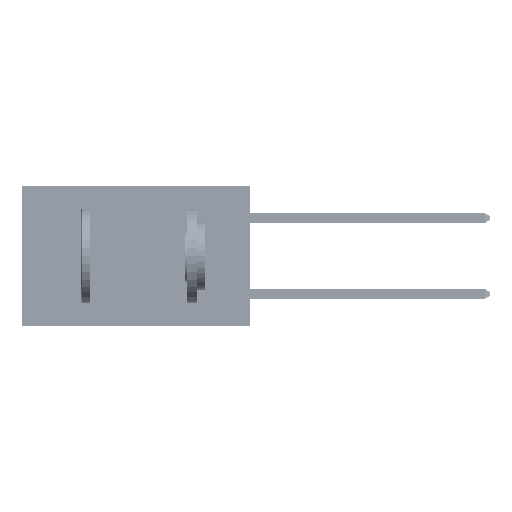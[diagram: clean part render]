
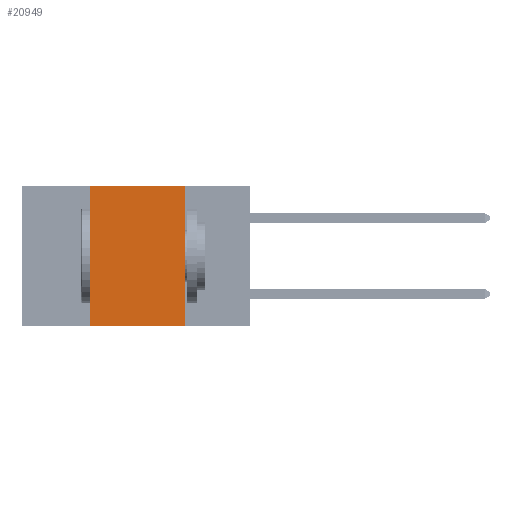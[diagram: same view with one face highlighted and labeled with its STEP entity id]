
A CAD part, left-side view. The second image highlights one B-rep face of the part: STEP entity #20949.
In plain terms, the highlighted planar face has unit normal (-1, 0, 0).
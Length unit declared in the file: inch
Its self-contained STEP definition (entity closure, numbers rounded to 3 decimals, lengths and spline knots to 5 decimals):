
#704 = VECTOR ( 'NONE', #45560, 39.37008 ) ;
#7364 = CARTESIAN_POINT ( 'NONE',  ( 0., 0.6, 0. ) ) ;
#10146 = CARTESIAN_POINT ( 'NONE',  ( 0., 0.17, 0. ) ) ;
#11163 = VERTEX_POINT ( 'NONE', #21826 ) ;
#11632 = AXIS2_PLACEMENT_3D ( 'NONE', #7364, #15367, #20673 ) ;
#12358 = LINE ( 'NONE', #42086, #704 ) ;
#12411 = EDGE_CURVE ( 'NONE', #17411, #30723, #38642, .T. ) ;
#13023 = DIRECTION ( 'NONE',  ( 0., -1., 0. ) ) ;
#13771 = EDGE_LOOP ( 'NONE', ( #38287, #25829, #31517, #31889 ) ) ;
#14412 = LINE ( 'NONE', #19038, #44380 ) ;
#15367 = DIRECTION ( 'NONE',  ( 1., 0., 0. ) ) ;
#16229 = EDGE_CURVE ( 'NONE', #17411, #11163, #12358, .T. ) ;
#16359 = VERTEX_POINT ( 'NONE', #49490 ) ;
#17411 = VERTEX_POINT ( 'NONE', #23085 ) ;
#19038 = CARTESIAN_POINT ( 'NONE',  ( 0., 0.6, 0. ) ) ;
#20673 = DIRECTION ( 'NONE',  ( 0., 0., -1. ) ) ;
#20723 = CARTESIAN_POINT ( 'NONE',  ( 0., 0.6, -0.37 ) ) ;
#20949 = ADVANCED_FACE ( 'NONE', ( #33537 ), #26985, .F. ) ;
#21826 = CARTESIAN_POINT ( 'NONE',  ( 0., 0.42, 0. ) ) ;
#23085 = CARTESIAN_POINT ( 'NONE',  ( 0., 0.42, -0.37 ) ) ;
#25829 = ORIENTED_EDGE ( 'NONE', *, *, #42701, .F. ) ;
#26985 = PLANE ( 'NONE',  #11632 ) ;
#27587 = LINE ( 'NONE', #10146, #44094 ) ;
#30723 = VERTEX_POINT ( 'NONE', #49356 ) ;
#31517 = ORIENTED_EDGE ( 'NONE', *, *, #16229, .F. ) ;
#31889 = ORIENTED_EDGE ( 'NONE', *, *, #12411, .T. ) ;
#33537 = FACE_OUTER_BOUND ( 'NONE', #13771, .T. ) ;
#38287 = ORIENTED_EDGE ( 'NONE', *, *, #45279, .F. ) ;
#38642 = LINE ( 'NONE', #20723, #46609 ) ;
#42086 = CARTESIAN_POINT ( 'NONE',  ( 0., 0.42, 0. ) ) ;
#42373 = DIRECTION ( 'NONE',  ( 0., 0., -1. ) ) ;
#42701 = EDGE_CURVE ( 'NONE', #11163, #16359, #14412, .T. ) ;
#44094 = VECTOR ( 'NONE', #42373, 39.37008 ) ;
#44380 = VECTOR ( 'NONE', #45878, 39.37008 ) ;
#45279 = EDGE_CURVE ( 'NONE', #16359, #30723, #27587, .T. ) ;
#45560 = DIRECTION ( 'NONE',  ( 0., 0., 1. ) ) ;
#45878 = DIRECTION ( 'NONE',  ( 0., -1., 0. ) ) ;
#46609 = VECTOR ( 'NONE', #13023, 39.37008 ) ;
#49356 = CARTESIAN_POINT ( 'NONE',  ( 0., 0.17, -0.37 ) ) ;
#49490 = CARTESIAN_POINT ( 'NONE',  ( 0., 0.17, 0. ) ) ;
